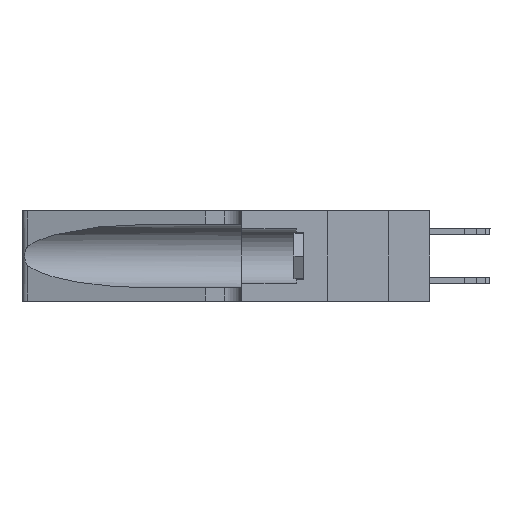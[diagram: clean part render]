
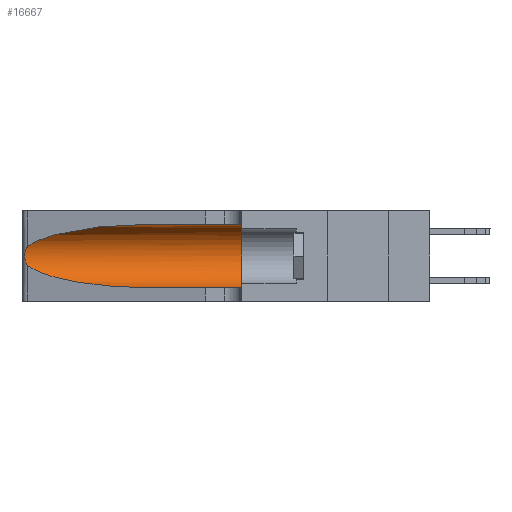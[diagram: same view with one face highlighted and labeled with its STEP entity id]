
A CAD part, left-side view. The second image highlights one B-rep face of the part: STEP entity #16667.
In plain terms, the highlighted cylindrical face has radius 3.308 mm (diameter 6.617 mm), a partial arc.
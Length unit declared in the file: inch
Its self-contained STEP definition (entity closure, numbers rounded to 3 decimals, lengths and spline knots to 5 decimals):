
#75 = CARTESIAN_POINT ( 'NONE',  ( 0.26075, 1.23896, 0.19203 ) ) ;
#158 = CARTESIAN_POINT ( 'NONE',  ( 0.25555, 1.22993, 0.14849 ) ) ;
#373 = CARTESIAN_POINT ( 'NONE',  ( 0.1305, 0.72297, 0.31525 ) ) ;
#648 = DIRECTION ( 'NONE',  ( 0., -1., 0. ) ) ;
#906 = VERTEX_POINT ( 'NONE', #373 ) ;
#932 = EDGE_LOOP ( 'NONE', ( #21036, #14998, #5735, #16379, #17875, #14462 ) ) ;
#934 = CARTESIAN_POINT ( 'NONE',  ( 0.18966, 0.96281, 0.31525 ) ) ;
#1132 = EDGE_CURVE ( 'NONE', #906, #11152, #7318, .T. ) ;
#2473 = CARTESIAN_POINT ( 'NONE',  ( 0.1305, 1.61858, 0.185 ) ) ;
#2482 = EDGE_CURVE ( 'NONE', #906, #4147, #8148, .T. ) ;
#2782 = EDGE_CURVE ( 'NONE', #15855, #22045, #4252, .T. ) ;
#3436 = CARTESIAN_POINT ( 'NONE',  ( 0.1305, 1.61858, 0.05475 ) ) ;
#3624 = B_SPLINE_CURVE_WITH_KNOTS ( 'NONE', 3,
 ( #7706, #21008, #11456, #5773, #19182, #17413, #75, #21158, #15386, #13538, #3943, #23069, #158, #11775 ),
 .UNSPECIFIED., .F., .F.,
 ( 4, 2, 2, 2, 2, 2, 4 ),
 ( 0., 0.00027, 0.00053, 0.00107, 0.0016, 0.00187, 0.00214 ),
 .UNSPECIFIED. ) ;
#3702 = CARTESIAN_POINT ( 'NONE',  ( 0.25487, 1.22718, 0.14631 ) ) ;
#3943 = CARTESIAN_POINT ( 'NONE',  ( 0.25789, 1.23486, 0.15765 ) ) ;
#4147 = VERTEX_POINT ( 'NONE', #18733 ) ;
#4252 = LINE ( 'NONE', #3436, #20733 ) ;
#4369 = CARTESIAN_POINT ( 'NONE',  ( 0.25487, 1.22718, 0.14631 ) ) ;
#4687 =( BOUNDED_CURVE ( )  B_SPLINE_CURVE ( 3, ( #3702, #11068, #9122, #11141 ),
 .UNSPECIFIED., .F., .F. ) 
 B_SPLINE_CURVE_WITH_KNOTS ( ( 4, 4 ),
 ( 3.44316, 4.71239 ),
 .UNSPECIFIED. ) 
 CURVE ( )  GEOMETRIC_REPRESENTATION_ITEM ( )  RATIONAL_B_SPLINE_CURVE ( ( 1., 0.87, 0.87, 1. ) ) 
 REPRESENTATION_ITEM ( '' )  );
#5542 = CARTESIAN_POINT ( 'NONE',  ( 0.1305, 0.72297, 0.05475 ) ) ;
#5735 = ORIENTED_EDGE ( 'NONE', *, *, #20907, .T. ) ;
#5773 = CARTESIAN_POINT ( 'NONE',  ( 0.25787, 1.23484, 0.2124 ) ) ;
#7318 =( BOUNDED_CURVE ( )  B_SPLINE_CURVE ( 3, ( #21981, #934, #12480, #8680 ),
 .UNSPECIFIED., .F., .F. ) 
 B_SPLINE_CURVE_WITH_KNOTS ( ( 4, 4 ),
 ( 1.5708, 2.84003 ),
 .UNSPECIFIED. ) 
 CURVE ( )  GEOMETRIC_REPRESENTATION_ITEM ( )  RATIONAL_B_SPLINE_CURVE ( ( 1., 0.87, 0.87, 1. ) ) 
 REPRESENTATION_ITEM ( '' )  );
#7579 = VECTOR ( 'NONE', #648, 39.37008 ) ;
#7706 = CARTESIAN_POINT ( 'NONE',  ( 0.25487, 1.22718, 0.22369 ) ) ;
#8148 = LINE ( 'NONE', #21539, #7579 ) ;
#8680 = CARTESIAN_POINT ( 'NONE',  ( 0.25487, 1.22718, 0.22369 ) ) ;
#9122 = CARTESIAN_POINT ( 'NONE',  ( 0.18966, 0.96281, 0.05475 ) ) ;
#10009 = DIRECTION ( 'NONE',  ( 0., -1., 0. ) ) ;
#10233 = DIRECTION ( 'NONE',  ( 0., 1., 0. ) ) ;
#10906 = EDGE_CURVE ( 'NONE', #4147, #22045, #18956, .T. ) ;
#10916 = CARTESIAN_POINT ( 'NONE',  ( 0.1305, 0.35, 0.05475 ) ) ;
#11068 = CARTESIAN_POINT ( 'NONE',  ( 0.2373, 1.15595, 0.08982 ) ) ;
#11141 = CARTESIAN_POINT ( 'NONE',  ( 0.1305, 0.72297, 0.05475 ) ) ;
#11152 = VERTEX_POINT ( 'NONE', #12024 ) ;
#11456 = CARTESIAN_POINT ( 'NONE',  ( 0.25639, 1.23184, 0.21858 ) ) ;
#11775 = CARTESIAN_POINT ( 'NONE',  ( 0.25487, 1.22718, 0.14631 ) ) ;
#12022 = VERTEX_POINT ( 'NONE', #4369 ) ;
#12024 = CARTESIAN_POINT ( 'NONE',  ( 0.25487, 1.22718, 0.22369 ) ) ;
#12342 = EDGE_CURVE ( 'NONE', #11152, #12022, #3624, .T. ) ;
#12460 = FACE_OUTER_BOUND ( 'NONE', #932, .T. ) ;
#12480 = CARTESIAN_POINT ( 'NONE',  ( 0.2373, 1.15595, 0.28018 ) ) ;
#13054 = DIRECTION ( 'NONE',  ( 0., -1., 0. ) ) ;
#13538 = CARTESIAN_POINT ( 'NONE',  ( 0.25856, 1.23593, 0.16098 ) ) ;
#13698 = DIRECTION ( 'NONE',  ( 0., 0., -1. ) ) ;
#14462 = ORIENTED_EDGE ( 'NONE', *, *, #2482, .F. ) ;
#14998 = ORIENTED_EDGE ( 'NONE', *, *, #12342, .T. ) ;
#15386 = CARTESIAN_POINT ( 'NONE',  ( 0.26017, 1.23833, 0.17102 ) ) ;
#15434 = CYLINDRICAL_SURFACE ( 'NONE', #21712, 0.13025 ) ;
#15855 = VERTEX_POINT ( 'NONE', #5542 ) ;
#16379 = ORIENTED_EDGE ( 'NONE', *, *, #2782, .T. ) ;
#16667 = ADVANCED_FACE ( 'NONE', ( #12460 ), #15434, .F. ) ;
#17413 = CARTESIAN_POINT ( 'NONE',  ( 0.26018, 1.23835, 0.19895 ) ) ;
#17696 = CARTESIAN_POINT ( 'NONE',  ( 0.1305, 0.35, 0.185 ) ) ;
#17767 = DIRECTION ( 'NONE',  ( 0., 0., 1. ) ) ;
#17875 = ORIENTED_EDGE ( 'NONE', *, *, #10906, .F. ) ;
#18733 = CARTESIAN_POINT ( 'NONE',  ( 0.1305, 0.35, 0.31525 ) ) ;
#18956 = CIRCLE ( 'NONE', #21791, 0.13025 ) ;
#19182 = CARTESIAN_POINT ( 'NONE',  ( 0.25854, 1.2359, 0.20912 ) ) ;
#20733 = VECTOR ( 'NONE', #13054, 39.37008 ) ;
#20907 = EDGE_CURVE ( 'NONE', #12022, #15855, #4687, .T. ) ;
#21008 = CARTESIAN_POINT ( 'NONE',  ( 0.25555, 1.22994, 0.2215 ) ) ;
#21036 = ORIENTED_EDGE ( 'NONE', *, *, #1132, .T. ) ;
#21158 = CARTESIAN_POINT ( 'NONE',  ( 0.26075, 1.23896, 0.178 ) ) ;
#21539 = CARTESIAN_POINT ( 'NONE',  ( 0.1305, 1.61858, 0.31525 ) ) ;
#21712 = AXIS2_PLACEMENT_3D ( 'NONE', #2473, #10009, #13698 ) ;
#21791 = AXIS2_PLACEMENT_3D ( 'NONE', #17696, #10233, #17767 ) ;
#21981 = CARTESIAN_POINT ( 'NONE',  ( 0.1305, 0.72297, 0.31525 ) ) ;
#22045 = VERTEX_POINT ( 'NONE', #10916 ) ;
#23069 = CARTESIAN_POINT ( 'NONE',  ( 0.25639, 1.23186, 0.15144 ) ) ;
